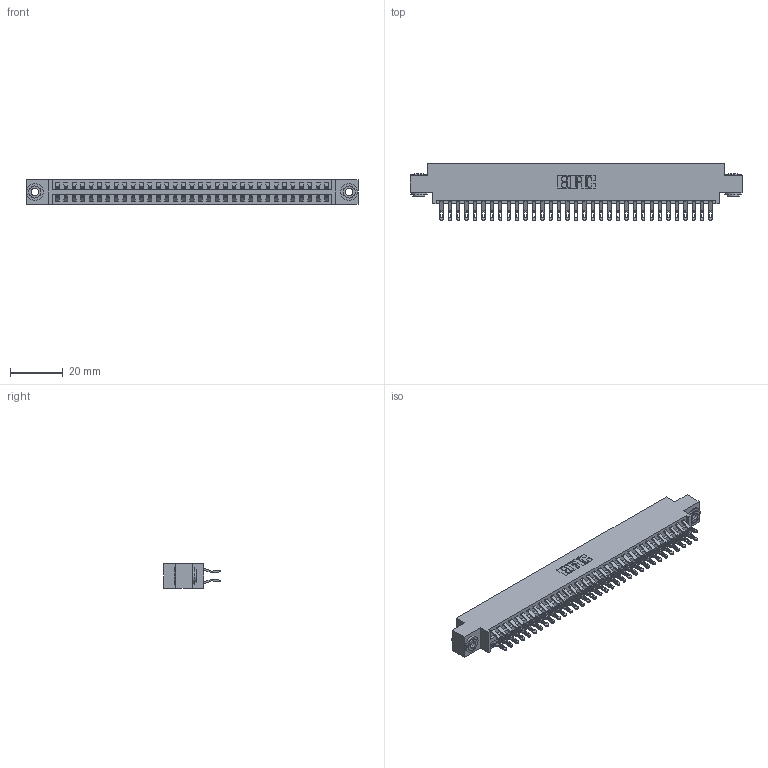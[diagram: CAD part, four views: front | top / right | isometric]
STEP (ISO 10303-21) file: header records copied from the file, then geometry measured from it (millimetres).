
FILE_DESCRIPTION (( 'STEP AP203' ), '1' );
FILE_NAME ('346-066-555-803.STEP', '2022-05-24T17:39:18', ( '' ), ( '' ), 'SwSTEP 2.0', 'SolidWorks 2020', '' );
FILE_SCHEMA (( 'CONFIG_CONTROL_DESIGN' ));
Length unit declared in the file: inch
Products named in the file (4): 346 Part_0.170 Offset - 0.156 Dia-TH; 346-066-555-803; 345-250-002_345-250-002-102; 345-292-001_555 Tail
Assembly tree (69 placements, depth 2):
  346-066-555-803
    346 Part_0.170 Offset - 0.156 Dia-TH
    345-292-001_555 Tail  x66
    345-250-002_345-250-002-102  x2
Bounding box: 125.35 x 21.46 x 9.4 mm (x, y, z)
Volume: 12191.3 mm3; surface area: 17727.1 mm2
Topology: 69 solids, 69 shells, 4006 faces, 12531 edges, 8350 vertices
Faces by surface type: plane 2282, cylinder 1716, cone 8
Entity records: 24272 total; most frequent: CARTESIAN_POINT 4031, ORIENTED_EDGE 3926, DIRECTION 3601, EDGE_CURVE 1963, LINE 1655, VECTOR 1655, VERTEX_POINT 1306, AXIS2_PLACEMENT_3D 973
